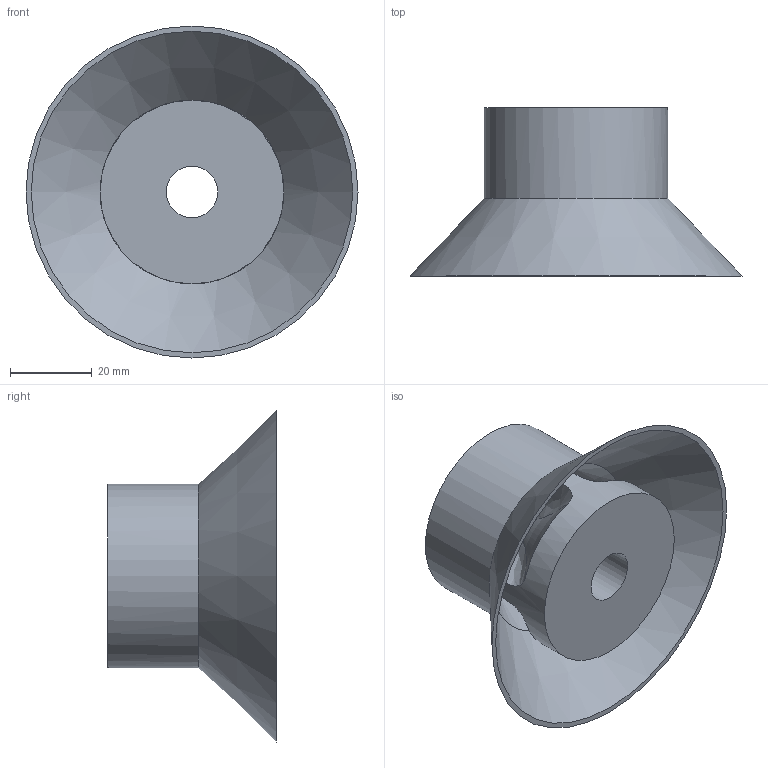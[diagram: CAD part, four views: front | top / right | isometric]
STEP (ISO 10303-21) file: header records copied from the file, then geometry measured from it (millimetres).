
FILE_DESCRIPTION(/* description */ (''),/* implementation_level */ '2;1');
FILE_NAME(/* name */ '1.77 Dia 50 CAL Baffle STEP.step',/* time_stamp */ '2019-06-01T15:58:54-04:00',/* author */ (''),/* organization */ (''),/* preprocessor_version */ 'ST-DEVELOPER v18',/* originating_system */ 'Autodesk Translation Framework v8.2.0.1029',/* authorisation */ '');
FILE_SCHEMA (('AUTOMOTIVE_DESIGN { 1 0 10303 214 3 1 1 }'));
Length unit declared in the file: inch
Products named in the file (1): 1.77 dia 1.624 high 50 cal
Bounding box: 81.28 x 41.25 x 81.28 mm (x, y, z)
Volume: 50235.7 mm3; surface area: 23920.2 mm2
Topology: 1 solids, 1 shells, 32 faces, 114 edges, 77 vertices
Faces by surface type: bspline 13, plane 11, cylinder 4, cone 2, torus 2
Full cylindrical faces by diameter (mm): 12.7 x2, 44.958 x2
Entity records: 1969 total; most frequent: CARTESIAN_POINT 1078, ORIENTED_EDGE 228, DIRECTION 120, EDGE_CURVE 114, VERTEX_POINT 77, B_SPLINE_CURVE_WITH_KNOTS 66, AXIS2_PLACEMENT_3D 53, EDGE_LOOP 35
